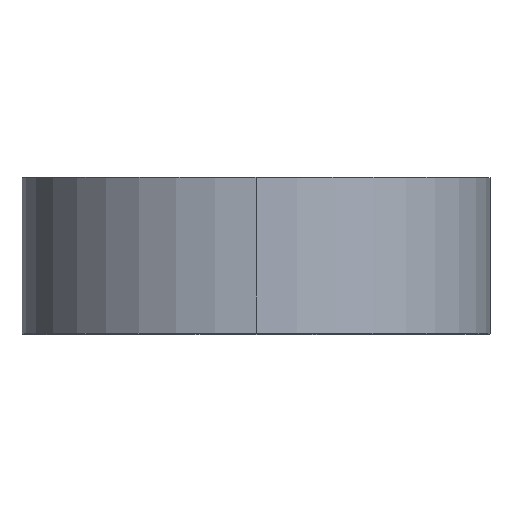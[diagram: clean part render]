
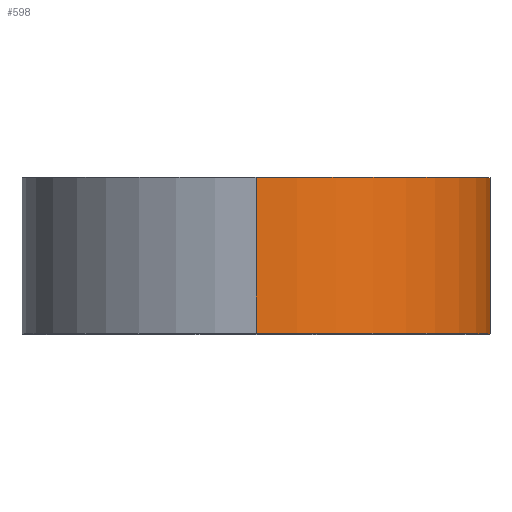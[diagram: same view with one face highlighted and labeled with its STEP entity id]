
A CAD part, top view. The second image highlights one B-rep face of the part: STEP entity #598.
In plain terms, the highlighted cylindrical face has radius 7.5 mm (diameter 15 mm), a partial arc.
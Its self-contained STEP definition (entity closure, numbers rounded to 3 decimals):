
#23 = DIRECTION ( 'NONE',  ( 0., 0., -1. ) ) ;
#68 = CIRCLE ( 'NONE', #461, 7.5 ) ;
#100 = CARTESIAN_POINT ( 'NONE',  ( 7.5, 2.5, 2.5 ) ) ;
#130 = VECTOR ( 'NONE', #1174, 1000. ) ;
#140 = LINE ( 'NONE', #475, #130 ) ;
#142 = DIRECTION ( 'NONE',  ( 0., -1., 0. ) ) ;
#217 = CIRCLE ( 'NONE', #631, 7.5 ) ;
#260 = CARTESIAN_POINT ( 'NONE',  ( 0., 2.5, 10. ) ) ;
#266 = CYLINDRICAL_SURFACE ( 'NONE', #636, 7.5 ) ;
#283 = FACE_OUTER_BOUND ( 'NONE', #1549, .T. ) ;
#347 = DIRECTION ( 'NONE',  ( 0., -1., 0. ) ) ;
#461 = AXIS2_PLACEMENT_3D ( 'NONE', #1489, #723, #23 ) ;
#475 = CARTESIAN_POINT ( 'NONE',  ( 7.5, -2.5, 2.5 ) ) ;
#598 = ADVANCED_FACE ( 'NONE', ( #283 ), #266, .T. ) ;
#631 = AXIS2_PLACEMENT_3D ( 'NONE', #1191, #347, #1318 ) ;
#633 = VERTEX_POINT ( 'NONE', #100 ) ;
#636 = AXIS2_PLACEMENT_3D ( 'NONE', #1516, #142, #1305 ) ;
#690 = VECTOR ( 'NONE', #1309, 1000. ) ;
#723 = DIRECTION ( 'NONE',  ( 0., 1., 0. ) ) ;
#820 = VERTEX_POINT ( 'NONE', #1482 ) ;
#862 = EDGE_CURVE ( 'NONE', #820, #1541, #217, .T. ) ;
#964 = LINE ( 'NONE', #1310, #690 ) ;
#972 = EDGE_CURVE ( 'NONE', #633, #820, #140, .T. ) ;
#1078 = CARTESIAN_POINT ( 'NONE',  ( 0., -2.5, 10. ) ) ;
#1079 = EDGE_CURVE ( 'NONE', #1277, #633, #68, .T. ) ;
#1174 = DIRECTION ( 'NONE',  ( 0., -1., 0. ) ) ;
#1185 = EDGE_CURVE ( 'NONE', #1541, #1277, #964, .T. ) ;
#1191 = CARTESIAN_POINT ( 'NONE',  ( 0., -2.5, 2.5 ) ) ;
#1277 = VERTEX_POINT ( 'NONE', #260 ) ;
#1305 = DIRECTION ( 'NONE',  ( 1., 0., 0. ) ) ;
#1309 = DIRECTION ( 'NONE',  ( 0., 1., 0. ) ) ;
#1310 = CARTESIAN_POINT ( 'NONE',  ( 0., 2.5, 10. ) ) ;
#1318 = DIRECTION ( 'NONE',  ( 0., 0., 1. ) ) ;
#1477 = ORIENTED_EDGE ( 'NONE', *, *, #972, .F. ) ;
#1478 = ORIENTED_EDGE ( 'NONE', *, *, #1079, .F. ) ;
#1479 = ORIENTED_EDGE ( 'NONE', *, *, #1185, .F. ) ;
#1480 = ORIENTED_EDGE ( 'NONE', *, *, #862, .F. ) ;
#1482 = CARTESIAN_POINT ( 'NONE',  ( 7.5, -2.5, 2.5 ) ) ;
#1489 = CARTESIAN_POINT ( 'NONE',  ( 0., 2.5, 2.5 ) ) ;
#1516 = CARTESIAN_POINT ( 'NONE',  ( 0., 0., 2.5 ) ) ;
#1541 = VERTEX_POINT ( 'NONE', #1078 ) ;
#1549 = EDGE_LOOP ( 'NONE', ( #1477, #1478, #1479, #1480 ) ) ;
